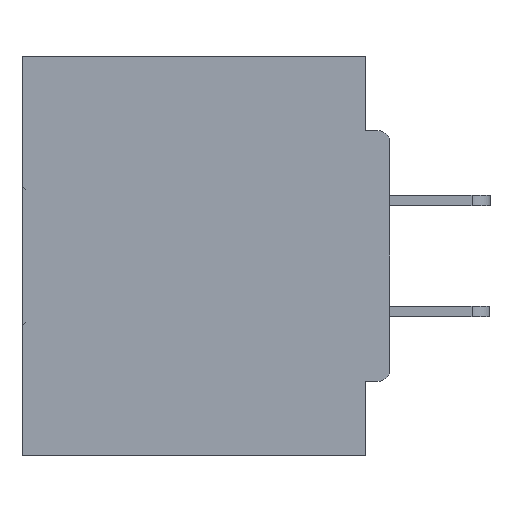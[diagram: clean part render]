
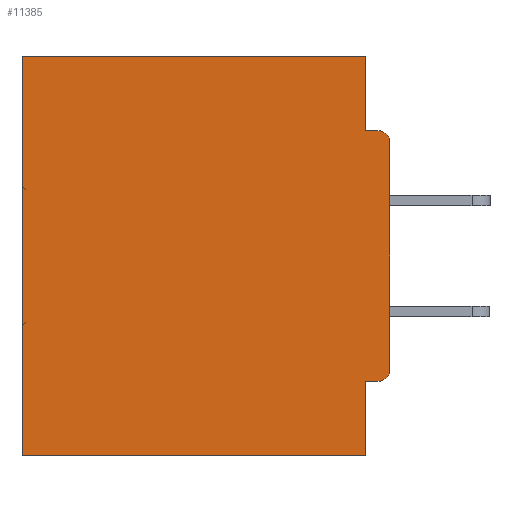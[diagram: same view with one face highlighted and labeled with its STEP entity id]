
A CAD part, left-side view. The second image highlights one B-rep face of the part: STEP entity #11385.
In plain terms, the highlighted planar face has unit normal (-1, 0, 0).
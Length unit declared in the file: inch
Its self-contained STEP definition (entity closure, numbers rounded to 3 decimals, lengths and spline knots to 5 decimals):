
#1018 = EDGE_CURVE ( 'NONE', #30674, #45405, #32798, .T. ) ;
#1053 = ORIENTED_EDGE ( 'NONE', *, *, #33641, .F. ) ;
#1470 = CARTESIAN_POINT ( 'NONE',  ( 0.298, 0., 0. ) ) ;
#1545 = EDGE_CURVE ( 'NONE', #15284, #13930, #34397, .T. ) ;
#1581 = DIRECTION ( 'NONE',  ( 0., 0., -1. ) ) ;
#2428 = ORIENTED_EDGE ( 'NONE', *, *, #34486, .F. ) ;
#3200 = ORIENTED_EDGE ( 'NONE', *, *, #36298, .T. ) ;
#3622 = ORIENTED_EDGE ( 'NONE', *, *, #1545, .F. ) ;
#4100 = ORIENTED_EDGE ( 'NONE', *, *, #41606, .T. ) ;
#4308 = EDGE_CURVE ( 'NONE', #45237, #16241, #15510, .T. ) ;
#4334 = CARTESIAN_POINT ( 'NONE',  ( 0.298, 0.46, 0. ) ) ;
#5157 = VERTEX_POINT ( 'NONE', #19974 ) ;
#5426 = ORIENTED_EDGE ( 'NONE', *, *, #1018, .F. ) ;
#6374 = CARTESIAN_POINT ( 'NONE',  ( 0.298, 0.031, 0. ) ) ;
#8073 = VERTEX_POINT ( 'NONE', #23167 ) ;
#8410 = DIRECTION ( 'NONE',  ( 1., 0., 0. ) ) ;
#8650 = VECTOR ( 'NONE', #26660, 39.37008 ) ;
#8901 = VECTOR ( 'NONE', #18663, 39.37008 ) ;
#11209 = ORIENTED_EDGE ( 'NONE', *, *, #19966, .F. ) ;
#11385 = ADVANCED_FACE ( 'NONE', ( #27748 ), #22583, .F. ) ;
#12272 = CARTESIAN_POINT ( 'NONE',  ( 0.298, 0.031, -0.4065 ) ) ;
#12913 = CIRCLE ( 'NONE', #21165, 0.015 ) ;
#13104 = LINE ( 'NONE', #15966, #8650 ) ;
#13228 = CARTESIAN_POINT ( 'NONE',  ( 0.298, 0., -0.1085 ) ) ;
#13605 = DIRECTION ( 'NONE',  ( 0., 0., -1. ) ) ;
#13898 = DIRECTION ( 'NONE',  ( 0., 0., -1. ) ) ;
#13917 = VERTEX_POINT ( 'NONE', #12272 ) ;
#13930 = VERTEX_POINT ( 'NONE', #28075 ) ;
#14329 = CARTESIAN_POINT ( 'NONE',  ( 0.298, 0.031, -0.5 ) ) ;
#14593 = LINE ( 'NONE', #38688, #20139 ) ;
#15179 = DIRECTION ( 'NONE',  ( 0., 0., -1. ) ) ;
#15247 = VERTEX_POINT ( 'NONE', #14329 ) ;
#15284 = VERTEX_POINT ( 'NONE', #13228 ) ;
#15419 = CARTESIAN_POINT ( 'NONE',  ( 0.298, 0., 0. ) ) ;
#15510 = LINE ( 'NONE', #1470, #39434 ) ;
#15966 = CARTESIAN_POINT ( 'NONE',  ( 0.298, 0.031, -0.5 ) ) ;
#16241 = VERTEX_POINT ( 'NONE', #4334 ) ;
#16603 = LINE ( 'NONE', #34917, #34429 ) ;
#17900 = CIRCLE ( 'NONE', #40197, 0.015 ) ;
#18377 = ORIENTED_EDGE ( 'NONE', *, *, #26809, .F. ) ;
#18663 = DIRECTION ( 'NONE',  ( 0., 0., -1. ) ) ;
#19966 = EDGE_CURVE ( 'NONE', #8073, #13917, #26061, .T. ) ;
#19974 = CARTESIAN_POINT ( 'NONE',  ( 0.298, 0.46, -0.5 ) ) ;
#20139 = VECTOR ( 'NONE', #28689, 39.37008 ) ;
#20297 = DIRECTION ( 'NONE',  ( 0., -1., 0. ) ) ;
#21165 = AXIS2_PLACEMENT_3D ( 'NONE', #35197, #42830, #13898 ) ;
#21380 = CARTESIAN_POINT ( 'NONE',  ( 0.298, 0.015, -0.3915 ) ) ;
#22583 = PLANE ( 'NONE',  #37859 ) ;
#23050 = ORIENTED_EDGE ( 'NONE', *, *, #4308, .T. ) ;
#23167 = CARTESIAN_POINT ( 'NONE',  ( 0.298, 0.015, -0.4065 ) ) ;
#23428 = DIRECTION ( 'NONE',  ( 0., 1., 0. ) ) ;
#24435 = CARTESIAN_POINT ( 'NONE',  ( 0.298, 0.015, -0.0935 ) ) ;
#24734 = VECTOR ( 'NONE', #1581, 39.37008 ) ;
#25583 = DIRECTION ( 'NONE',  ( 0., 0., -1. ) ) ;
#26061 = LINE ( 'NONE', #34034, #30535 ) ;
#26660 = DIRECTION ( 'NONE',  ( 0., 0., -1. ) ) ;
#26809 = EDGE_CURVE ( 'NONE', #15247, #5157, #14593, .T. ) ;
#27227 = VECTOR ( 'NONE', #20297, 39.37008 ) ;
#27748 = FACE_OUTER_BOUND ( 'NONE', #31749, .T. ) ;
#28075 = CARTESIAN_POINT ( 'NONE',  ( 0.298, 0., -0.3915 ) ) ;
#28689 = DIRECTION ( 'NONE',  ( 0., 1., 0. ) ) ;
#29792 = EDGE_CURVE ( 'NONE', #16241, #5157, #16603, .T. ) ;
#29819 = DIRECTION ( 'NONE',  ( 0., 1., 0. ) ) ;
#30388 = ORIENTED_EDGE ( 'NONE', *, *, #29792, .T. ) ;
#30535 = VECTOR ( 'NONE', #23428, 39.37008 ) ;
#30674 = VERTEX_POINT ( 'NONE', #34492 ) ;
#30933 = LINE ( 'NONE', #37285, #24734 ) ;
#31749 = EDGE_LOOP ( 'NONE', ( #4100, #5426, #1053, #23050, #30388, #18377, #2428, #11209, #3200, #3622 ) ) ;
#32636 = DIRECTION ( 'NONE',  ( -1., 0., 0. ) ) ;
#32798 = LINE ( 'NONE', #38094, #27227 ) ;
#33075 = CARTESIAN_POINT ( 'NONE',  ( 0.298, 0., 0. ) ) ;
#33641 = EDGE_CURVE ( 'NONE', #45237, #30674, #30933, .T. ) ;
#34034 = CARTESIAN_POINT ( 'NONE',  ( 0.298, 0., -0.4065 ) ) ;
#34397 = LINE ( 'NONE', #15419, #8901 ) ;
#34429 = VECTOR ( 'NONE', #13605, 39.37008 ) ;
#34486 = EDGE_CURVE ( 'NONE', #13917, #15247, #13104, .T. ) ;
#34492 = CARTESIAN_POINT ( 'NONE',  ( 0.298, 0.031, -0.0935 ) ) ;
#34917 = CARTESIAN_POINT ( 'NONE',  ( 0.298, 0.46, 0. ) ) ;
#35197 = CARTESIAN_POINT ( 'NONE',  ( 0.298, 0.015, -0.1085 ) ) ;
#36298 = EDGE_CURVE ( 'NONE', #8073, #13930, #17900, .T. ) ;
#37285 = CARTESIAN_POINT ( 'NONE',  ( 0.298, 0.031, -0.5 ) ) ;
#37859 = AXIS2_PLACEMENT_3D ( 'NONE', #33075, #8410, #15179 ) ;
#38094 = CARTESIAN_POINT ( 'NONE',  ( 0.298, 0., -0.0935 ) ) ;
#38688 = CARTESIAN_POINT ( 'NONE',  ( 0.298, 0., -0.5 ) ) ;
#39434 = VECTOR ( 'NONE', #29819, 39.37008 ) ;
#40197 = AXIS2_PLACEMENT_3D ( 'NONE', #21380, #32636, #25583 ) ;
#41606 = EDGE_CURVE ( 'NONE', #15284, #45405, #12913, .T. ) ;
#42830 = DIRECTION ( 'NONE',  ( -1., 0., 0. ) ) ;
#45237 = VERTEX_POINT ( 'NONE', #6374 ) ;
#45405 = VERTEX_POINT ( 'NONE', #24435 ) ;
